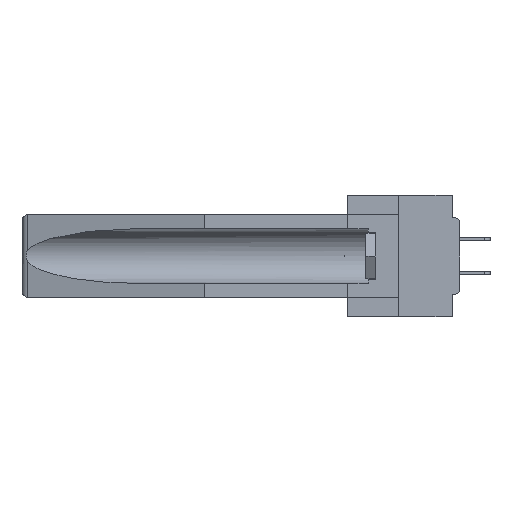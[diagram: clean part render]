
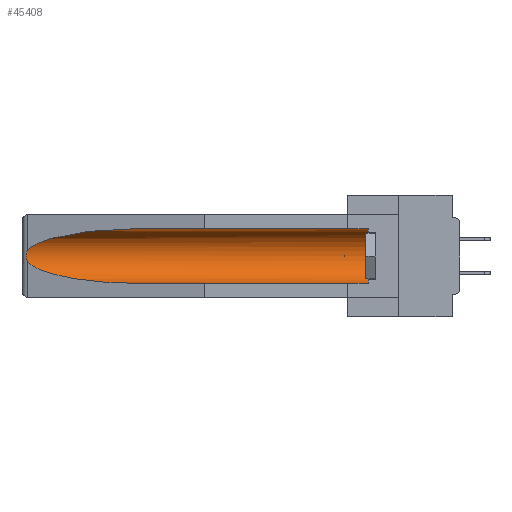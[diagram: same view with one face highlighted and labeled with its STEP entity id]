
A CAD part, left-side view. The second image highlights one B-rep face of the part: STEP entity #45408.
In plain terms, the highlighted cylindrical face has radius 2.857 mm (diameter 5.715 mm), a partial arc.
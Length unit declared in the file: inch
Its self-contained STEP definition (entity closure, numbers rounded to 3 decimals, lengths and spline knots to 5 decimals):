
#754 = ORIENTED_EDGE ( 'NONE', *, *, #40748, .T. ) ;
#1789 = CARTESIAN_POINT ( 'NONE',  ( 0.26597, 1.52961, -0.15275 ) ) ;
#2016 = DIRECTION ( 'NONE',  ( 0., 1., 0. ) ) ;
#2944 = VERTEX_POINT ( 'NONE', #46473 ) ;
#3109 = CARTESIAN_POINT ( 'NONE',  ( 0.155, -0.30754, -0.1715 ) ) ;
#3549 = VECTOR ( 'NONE', #43897, 39.37008 ) ;
#4678 = EDGE_CURVE ( 'NONE', #26372, #40347, #14506, .T. ) ;
#5636 = CARTESIAN_POINT ( 'NONE',  ( 0.26597, 1.5296, -0.19026 ) ) ;
#5791 = CARTESIAN_POINT ( 'NONE',  ( 0.26654, 1.53092, -0.15636 ) ) ;
#6522 = FACE_OUTER_BOUND ( 'NONE', #35331, .T. ) ;
#6765 = DIRECTION ( 'NONE',  ( 0., 1., 0. ) ) ;
#6867 = CARTESIAN_POINT ( 'NONE',  ( 0.26537, 1.52718, -0.19328 ) ) ;
#7185 = CARTESIAN_POINT ( 'NONE',  ( 0.25451, 1.48313, -0.24835 ) ) ;
#9652 =( BOUNDED_CURVE ( )  B_SPLINE_CURVE ( 3, ( #6867, #7185, #10941, #25607 ),
 .UNSPECIFIED., .F., .F. ) 
 B_SPLINE_CURVE_WITH_KNOTS ( ( 4, 4 ),
 ( 0.1948, 1.5708 ),
 .UNSPECIFIED. ) 
 CURVE ( )  GEOMETRIC_REPRESENTATION_ITEM ( )  RATIONAL_B_SPLINE_CURVE ( ( 1., 0.848, 0.848, 1. ) ) 
 REPRESENTATION_ITEM ( '' )  );
#10941 = CARTESIAN_POINT ( 'NONE',  ( 0.21114, 1.30732, -0.284 ) ) ;
#11261 = DIRECTION ( 'NONE',  ( 0., 0., 1. ) ) ;
#12858 = ORIENTED_EDGE ( 'NONE', *, *, #44204, .T. ) ;
#14506 = LINE ( 'NONE', #33244, #3549 ) ;
#14621 = VERTEX_POINT ( 'NONE', #23903 ) ;
#15479 = EDGE_CURVE ( 'NONE', #25916, #29034, #35368, .T. ) ;
#16513 = EDGE_CURVE ( 'NONE', #14621, #2944, #17861, .T. ) ;
#17256 = CARTESIAN_POINT ( 'NONE',  ( 0.25451, 1.48313, -0.09465 ) ) ;
#17861 = LINE ( 'NONE', #45741, #38643 ) ;
#18681 = CARTESIAN_POINT ( 'NONE',  ( 0.155, 0.126, -0.1715 ) ) ;
#20772 = ORIENTED_EDGE ( 'NONE', *, *, #16513, .T. ) ;
#23903 = CARTESIAN_POINT ( 'NONE',  ( 0.155, 0.126, -0.059 ) ) ;
#25607 = CARTESIAN_POINT ( 'NONE',  ( 0.155, 1.07973, -0.284 ) ) ;
#25916 = VERTEX_POINT ( 'NONE', #37033 ) ;
#26372 = VERTEX_POINT ( 'NONE', #47191 ) ;
#27615 = CARTESIAN_POINT ( 'NONE',  ( 0.2673, 1.5327, -0.16383 ) ) ;
#27617 = ORIENTED_EDGE ( 'NONE', *, *, #15479, .T. ) ;
#27706 = AXIS2_PLACEMENT_3D ( 'NONE', #3109, #6765, #43581 ) ;
#27773 = CARTESIAN_POINT ( 'NONE',  ( 0.26655, 1.53094, -0.18657 ) ) ;
#28712 = CARTESIAN_POINT ( 'NONE',  ( 0.155, 1.07973, -0.059 ) ) ;
#29034 = VERTEX_POINT ( 'NONE', #31339 ) ;
#29654 = DIRECTION ( 'NONE',  ( 0., -1., 0. ) ) ;
#30960 = CIRCLE ( 'NONE', #34744, 0.1125 ) ;
#31316 = CARTESIAN_POINT ( 'NONE',  ( 0.2673, 1.53269, -0.17917 ) ) ;
#31339 = CARTESIAN_POINT ( 'NONE',  ( 0.26537, 1.52718, -0.19328 ) ) ;
#31472 = CARTESIAN_POINT ( 'NONE',  ( 0.26537, 1.52718, -0.19328 ) ) ;
#31841 =( BOUNDED_CURVE ( )  B_SPLINE_CURVE ( 3, ( #28712, #43060, #17256, #32262 ),
 .UNSPECIFIED., .F., .F. ) 
 B_SPLINE_CURVE_WITH_KNOTS ( ( 4, 4 ),
 ( 4.71239, 6.08839 ),
 .UNSPECIFIED. ) 
 CURVE ( )  GEOMETRIC_REPRESENTATION_ITEM ( )  RATIONAL_B_SPLINE_CURVE ( ( 1., 0.848, 0.848, 1. ) ) 
 REPRESENTATION_ITEM ( '' )  );
#32262 = CARTESIAN_POINT ( 'NONE',  ( 0.26537, 1.52718, -0.14972 ) ) ;
#32893 = ORIENTED_EDGE ( 'NONE', *, *, #47249, .T. ) ;
#33244 = CARTESIAN_POINT ( 'NONE',  ( 0.155, -0.30754, -0.284 ) ) ;
#34744 = AXIS2_PLACEMENT_3D ( 'NONE', #18681, #29654, #11261 ) ;
#35322 = CARTESIAN_POINT ( 'NONE',  ( 0.2675, 1.53308, -0.17534 ) ) ;
#35331 = EDGE_LOOP ( 'NONE', ( #32893, #27617, #754, #47296, #12858, #20772 ) ) ;
#35368 = B_SPLINE_CURVE_WITH_KNOTS ( 'NONE', 3,
 ( #35622, #1789, #5791, #27615, #42600, #35322, #31316, #27773, #5636, #31472 ),
 .UNSPECIFIED., .F., .F.,
 ( 4, 2, 2, 2, 4 ),
 ( 0., 0.00029, 0.00058, 0.00087, 0.00117 ),
 .UNSPECIFIED. ) ;
#35622 = CARTESIAN_POINT ( 'NONE',  ( 0.26537, 1.52718, -0.14972 ) ) ;
#37033 = CARTESIAN_POINT ( 'NONE',  ( 0.26537, 1.52718, -0.14972 ) ) ;
#38643 = VECTOR ( 'NONE', #2016, 39.37008 ) ;
#39456 = CYLINDRICAL_SURFACE ( 'NONE', #27706, 0.1125 ) ;
#40347 = VERTEX_POINT ( 'NONE', #44865 ) ;
#40748 = EDGE_CURVE ( 'NONE', #29034, #40347, #9652, .T. ) ;
#42600 = CARTESIAN_POINT ( 'NONE',  ( 0.2675, 1.53308, -0.16763 ) ) ;
#43060 = CARTESIAN_POINT ( 'NONE',  ( 0.21114, 1.30732, -0.059 ) ) ;
#43581 = DIRECTION ( 'NONE',  ( 0., 0., 1. ) ) ;
#43897 = DIRECTION ( 'NONE',  ( 0., 1., 0. ) ) ;
#44204 = EDGE_CURVE ( 'NONE', #26372, #14621, #30960, .T. ) ;
#44865 = CARTESIAN_POINT ( 'NONE',  ( 0.155, 1.07973, -0.284 ) ) ;
#45408 = ADVANCED_FACE ( 'NONE', ( #6522 ), #39456, .F. ) ;
#45741 = CARTESIAN_POINT ( 'NONE',  ( 0.155, -0.30754, -0.059 ) ) ;
#46473 = CARTESIAN_POINT ( 'NONE',  ( 0.155, 1.07973, -0.059 ) ) ;
#47191 = CARTESIAN_POINT ( 'NONE',  ( 0.155, 0.126, -0.284 ) ) ;
#47249 = EDGE_CURVE ( 'NONE', #2944, #25916, #31841, .T. ) ;
#47296 = ORIENTED_EDGE ( 'NONE', *, *, #4678, .F. ) ;
